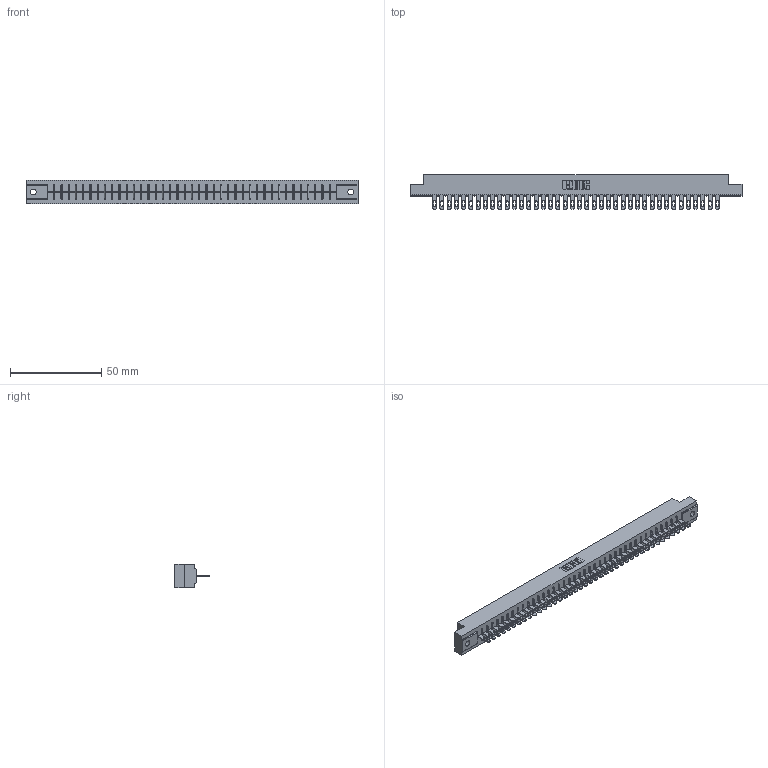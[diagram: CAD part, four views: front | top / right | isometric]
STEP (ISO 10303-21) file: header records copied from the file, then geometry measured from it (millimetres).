
FILE_DESCRIPTION (( 'STEP AP203' ), '1' );
FILE_NAME ('316-040-400-102.STEP', '2020-09-23T06:30:52', ( '' ), ( '' ), 'SwSTEP 2.0', 'SolidWorks 2020', '' );
FILE_SCHEMA (( 'CONFIG_CONTROL_DESIGN' ));
Length unit declared in the file: inch
Products named in the file (3): 316-040-400-102; 306 Part_.128 Dia; 306-290-001_100
Assembly tree (41 placements, depth 2):
  316-040-400-102
    306 Part_.128 Dia
    306-290-001_100  x40
Bounding box: 181.51 x 18.87 x 12.7 mm (x, y, z)
Volume: 20154.3 mm3; surface area: 21080.5 mm2
Topology: 41 solids, 41 shells, 3156 faces, 8916 edges, 5728 vertices
Faces by surface type: plane 2068, cylinder 928, sphere 160
Entity records: 37727 total; most frequent: CARTESIAN_POINT 6335, ORIENTED_EDGE 6280, DIRECTION 6248, EDGE_CURVE 3140, VECTOR 2454, LINE 2454, VERTEX_POINT 1984, AXIS2_PLACEMENT_3D 1897
